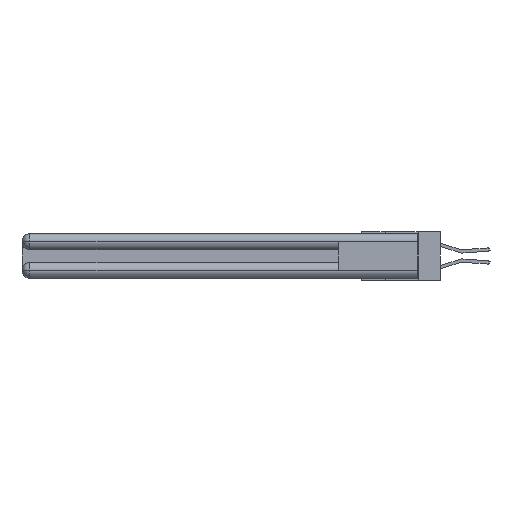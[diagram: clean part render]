
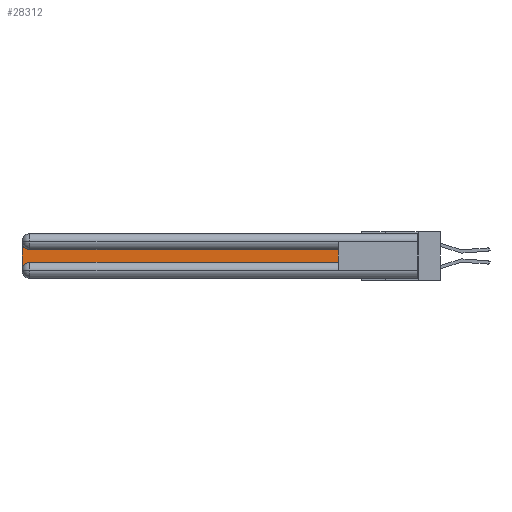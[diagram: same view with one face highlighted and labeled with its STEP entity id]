
A CAD part, left-side view. The second image highlights one B-rep face of the part: STEP entity #28312.
In plain terms, the highlighted planar face has unit normal (-1, 0, 0).
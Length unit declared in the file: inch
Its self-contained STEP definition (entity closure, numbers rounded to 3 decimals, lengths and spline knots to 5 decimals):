
#1116 = VECTOR ( 'NONE', #8655, 39.37008 ) ;
#1784 = EDGE_CURVE ( 'NONE', #23359, #33198, #10889, .T. ) ;
#2665 = AXIS2_PLACEMENT_3D ( 'NONE', #23522, #7775, #10279 ) ;
#3094 = CIRCLE ( 'NONE', #22948, 0.06 ) ;
#3600 = CARTESIAN_POINT ( 'NONE',  ( 0.075, 3., -0.1225 ) ) ;
#3892 = VERTEX_POINT ( 'NONE', #23950 ) ;
#4239 = DIRECTION ( 'NONE',  ( 0., -1., 0. ) ) ;
#4420 = DIRECTION ( 'NONE',  ( 0., 0., -1. ) ) ;
#4568 = EDGE_CURVE ( 'NONE', #5597, #17169, #3094, .T. ) ;
#5339 = VERTEX_POINT ( 'NONE', #26342 ) ;
#5597 = VERTEX_POINT ( 'NONE', #21924 ) ;
#5686 = EDGE_LOOP ( 'NONE', ( #23932, #23814, #9286, #15614, #27234, #31066 ) ) ;
#6559 = CIRCLE ( 'NONE', #2665, 0.06 ) ;
#7775 = DIRECTION ( 'NONE',  ( 1., 0., 0. ) ) ;
#8655 = DIRECTION ( 'NONE',  ( 0., 1., 0. ) ) ;
#8772 = CARTESIAN_POINT ( 'NONE',  ( 0.075, 0.6, -0.1225 ) ) ;
#9286 = ORIENTED_EDGE ( 'NONE', *, *, #12366, .T. ) ;
#9388 = EDGE_CURVE ( 'NONE', #5339, #23359, #6559, .T. ) ;
#10279 = DIRECTION ( 'NONE',  ( 0., 0., -1. ) ) ;
#10889 = LINE ( 'NONE', #22214, #31981 ) ;
#12303 = DIRECTION ( 'NONE',  ( 0., 0., -1. ) ) ;
#12366 = EDGE_CURVE ( 'NONE', #17169, #5339, #14838, .T. ) ;
#12382 = VECTOR ( 'NONE', #4420, 39.37008 ) ;
#13886 = DIRECTION ( 'NONE',  ( 1., 0., 0. ) ) ;
#14040 = CARTESIAN_POINT ( 'NONE',  ( 0.075, 0.6, -0.2175 ) ) ;
#14838 = LINE ( 'NONE', #32801, #12382 ) ;
#15614 = ORIENTED_EDGE ( 'NONE', *, *, #9388, .T. ) ;
#16775 = CARTESIAN_POINT ( 'NONE',  ( 0.075, 0.6, -0.2175 ) ) ;
#17169 = VERTEX_POINT ( 'NONE', #25683 ) ;
#17655 = FACE_OUTER_BOUND ( 'NONE', #5686, .T. ) ;
#18591 = AXIS2_PLACEMENT_3D ( 'NONE', #3600, #13886, #21898 ) ;
#21725 = EDGE_CURVE ( 'NONE', #3892, #5597, #28648, .T. ) ;
#21898 = DIRECTION ( 'NONE',  ( 0., 0., -1. ) ) ;
#21924 = CARTESIAN_POINT ( 'NONE',  ( 0.075, 2.94, -0.1225 ) ) ;
#22214 = CARTESIAN_POINT ( 'NONE',  ( 0.075, 0.6, -0.2175 ) ) ;
#22918 = CARTESIAN_POINT ( 'NONE',  ( 0.075, 2.94, -0.0625 ) ) ;
#22948 = AXIS2_PLACEMENT_3D ( 'NONE', #22918, #30188, #12303 ) ;
#23359 = VERTEX_POINT ( 'NONE', #24915 ) ;
#23522 = CARTESIAN_POINT ( 'NONE',  ( 0.075, 2.94, -0.2775 ) ) ;
#23814 = ORIENTED_EDGE ( 'NONE', *, *, #4568, .T. ) ;
#23932 = ORIENTED_EDGE ( 'NONE', *, *, #21725, .T. ) ;
#23950 = CARTESIAN_POINT ( 'NONE',  ( 0.075, 0.6, -0.1225 ) ) ;
#24915 = CARTESIAN_POINT ( 'NONE',  ( 0.075, 2.94, -0.2175 ) ) ;
#25683 = CARTESIAN_POINT ( 'NONE',  ( 0.075, 3., -0.0625 ) ) ;
#26342 = CARTESIAN_POINT ( 'NONE',  ( 0.075, 3., -0.2775 ) ) ;
#26692 = PLANE ( 'NONE',  #18591 ) ;
#27234 = ORIENTED_EDGE ( 'NONE', *, *, #1784, .T. ) ;
#28312 = ADVANCED_FACE ( 'NONE', ( #17655 ), #26692, .F. ) ;
#28648 = LINE ( 'NONE', #8772, #1116 ) ;
#28918 = VECTOR ( 'NONE', #29758, 39.37008 ) ;
#29736 = LINE ( 'NONE', #16775, #28918 ) ;
#29758 = DIRECTION ( 'NONE',  ( 0., 0., 1. ) ) ;
#30188 = DIRECTION ( 'NONE',  ( 1., 0., 0. ) ) ;
#31066 = ORIENTED_EDGE ( 'NONE', *, *, #33225, .T. ) ;
#31981 = VECTOR ( 'NONE', #4239, 39.37008 ) ;
#32801 = CARTESIAN_POINT ( 'NONE',  ( 0.075, 3., -0.2175 ) ) ;
#33198 = VERTEX_POINT ( 'NONE', #14040 ) ;
#33225 = EDGE_CURVE ( 'NONE', #33198, #3892, #29736, .T. ) ;
